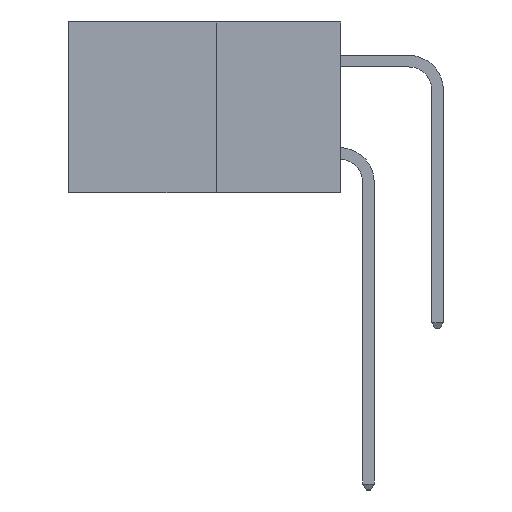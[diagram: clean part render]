
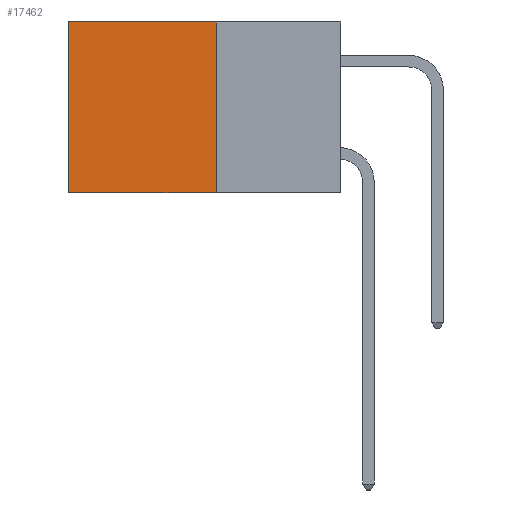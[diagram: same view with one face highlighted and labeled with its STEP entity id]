
A CAD part, left-side view. The second image highlights one B-rep face of the part: STEP entity #17462.
In plain terms, the highlighted planar face has unit normal (-1, 0, 0).
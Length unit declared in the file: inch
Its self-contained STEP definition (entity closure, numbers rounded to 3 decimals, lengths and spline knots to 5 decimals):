
#484 = VECTOR ( 'NONE', #3027, 39.37008 ) ;
#1221 = CARTESIAN_POINT ( 'NONE',  ( 0.277, 0.27, -0.37 ) ) ;
#1445 = CARTESIAN_POINT ( 'NONE',  ( 0.277, 0.27, -0.37 ) ) ;
#2355 = LINE ( 'NONE', #18622, #5856 ) ;
#3027 = DIRECTION ( 'NONE',  ( 0., 1., 0. ) ) ;
#3055 = VERTEX_POINT ( 'NONE', #10710 ) ;
#3342 = VERTEX_POINT ( 'NONE', #4994 ) ;
#3777 = PLANE ( 'NONE',  #11776 ) ;
#4994 = CARTESIAN_POINT ( 'NONE',  ( 0.277, 0.27, -0.37 ) ) ;
#5292 = DIRECTION ( 'NONE',  ( 1., 0., 0. ) ) ;
#5502 = VECTOR ( 'NONE', #12790, 39.37008 ) ;
#5612 = LINE ( 'NONE', #1445, #15813 ) ;
#5856 = VECTOR ( 'NONE', #9859, 39.37008 ) ;
#6109 = CARTESIAN_POINT ( 'NONE',  ( 0.277, 0.59, 0. ) ) ;
#6289 = FACE_OUTER_BOUND ( 'NONE', #11391, .T. ) ;
#6516 = VERTEX_POINT ( 'NONE', #6109 ) ;
#7576 = EDGE_CURVE ( 'NONE', #3055, #3342, #13183, .T. ) ;
#8825 = DIRECTION ( 'NONE',  ( 0., 1., 0. ) ) ;
#9198 = CARTESIAN_POINT ( 'NONE',  ( 0.277, 0.59, -0.37 ) ) ;
#9628 = EDGE_CURVE ( 'NONE', #3055, #6516, #16063, .T. ) ;
#9859 = DIRECTION ( 'NONE',  ( 0., 0., -1. ) ) ;
#10258 = EDGE_CURVE ( 'NONE', #3342, #11663, #5612, .T. ) ;
#10710 = CARTESIAN_POINT ( 'NONE',  ( 0.277, 0.27, 0. ) ) ;
#11391 = EDGE_LOOP ( 'NONE', ( #16589, #14835, #16640, #18461 ) ) ;
#11663 = VERTEX_POINT ( 'NONE', #9198 ) ;
#11776 = AXIS2_PLACEMENT_3D ( 'NONE', #13990, #5292, #15440 ) ;
#12790 = DIRECTION ( 'NONE',  ( 0., 0., -1. ) ) ;
#13183 = LINE ( 'NONE', #1221, #5502 ) ;
#13990 = CARTESIAN_POINT ( 'NONE',  ( 0.277, 0.27, -0.37 ) ) ;
#14729 = CARTESIAN_POINT ( 'NONE',  ( 0.277, 0.27, 0. ) ) ;
#14835 = ORIENTED_EDGE ( 'NONE', *, *, #10258, .F. ) ;
#15440 = DIRECTION ( 'NONE',  ( 0., 0., -1. ) ) ;
#15813 = VECTOR ( 'NONE', #8825, 39.37008 ) ;
#16063 = LINE ( 'NONE', #14729, #484 ) ;
#16589 = ORIENTED_EDGE ( 'NONE', *, *, #17059, .T. ) ;
#16640 = ORIENTED_EDGE ( 'NONE', *, *, #7576, .F. ) ;
#17059 = EDGE_CURVE ( 'NONE', #6516, #11663, #2355, .T. ) ;
#17462 = ADVANCED_FACE ( 'NONE', ( #6289 ), #3777, .F. ) ;
#18461 = ORIENTED_EDGE ( 'NONE', *, *, #9628, .T. ) ;
#18622 = CARTESIAN_POINT ( 'NONE',  ( 0.277, 0.59, -0.37 ) ) ;
